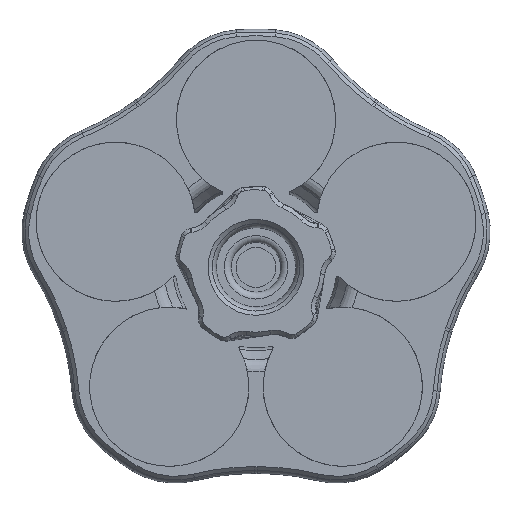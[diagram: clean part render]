
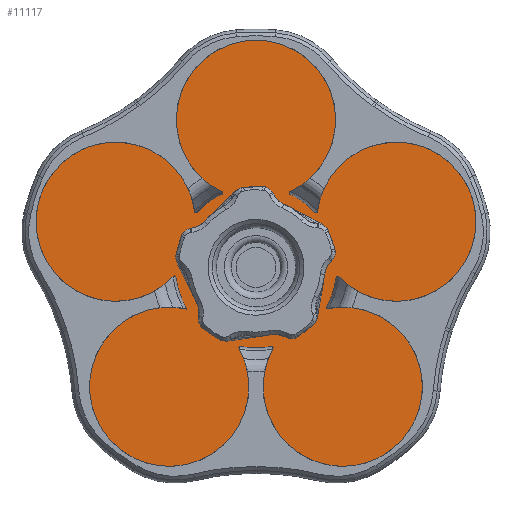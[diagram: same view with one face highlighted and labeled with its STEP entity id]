
A CAD part, front view. The second image highlights one B-rep face of the part: STEP entity #11117.
In plain terms, the highlighted planar face has unit normal (0, -1, 0).
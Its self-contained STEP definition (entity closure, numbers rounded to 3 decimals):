
#48=FACE_BOUND('',#3293,.T.);
#1013=CIRCLE('',#11928,0.1);
#1017=CIRCLE('',#11933,5.775);
#1022=CIRCLE('',#11940,0.1);
#1023=CIRCLE('',#11942,5.775);
#1027=CIRCLE('',#11947,0.1);
#1029=CIRCLE('',#11950,0.1);
#1031=CIRCLE('',#11953,5.85);
#1038=CIRCLE('',#11964,5.775);
#1046=CIRCLE('',#11981,5.775);
#1050=CIRCLE('',#11986,0.1);
#1054=CIRCLE('',#11992,0.1);
#1060=CIRCLE('',#12003,0.1);
#1062=CIRCLE('',#12006,5.85);
#1064=CIRCLE('',#12009,0.1);
#1069=CIRCLE('',#12016,0.1);
#1071=CIRCLE('',#12019,5.775);
#1277=CIRCLE('',#12376,4.65);
#1281=CIRCLE('',#12384,5.85);
#1284=CIRCLE('',#12391,5.85);
#1286=CIRCLE('',#12395,5.85);
#2554=FACE_OUTER_BOUND('',#3292,.T.);
#3292=EDGE_LOOP('',(#9654,#9655,#9656,#9657,#9658,#9659,#9660,#9661,#9662,
#9663,#9664,#9665,#9666,#9667,#9668,#9669,#9670,#9671,#9672));
#3293=EDGE_LOOP('',(#9673));
#4805=VERTEX_POINT('',#22344);
#4806=VERTEX_POINT('',#22346);
#4822=VERTEX_POINT('',#22420);
#4826=VERTEX_POINT('',#22432);
#4827=VERTEX_POINT('',#22434);
#4828=VERTEX_POINT('',#22438);
#4844=VERTEX_POINT('',#22512);
#4847=VERTEX_POINT('',#22519);
#4848=VERTEX_POINT('',#22521);
#4870=VERTEX_POINT('',#22667);
#4889=VERTEX_POINT('',#22814);
#4890=VERTEX_POINT('',#22816);
#4902=VERTEX_POINT('',#22872);
#4904=VERTEX_POINT('',#22881);
#4916=VERTEX_POINT('',#22952);
#4917=VERTEX_POINT('',#22954);
#4919=VERTEX_POINT('',#22963);
#4923=VERTEX_POINT('',#22975);
#4924=VERTEX_POINT('',#22977);
#5091=VERTEX_POINT('',#23862);
#6151=EDGE_CURVE('',#4805,#4806,#1013,.F.);
#6169=EDGE_CURVE('',#4805,#4822,#1017,.T.);
#6175=EDGE_CURVE('',#4826,#4827,#1022,.F.);
#6177=EDGE_CURVE('',#4828,#4827,#1023,.T.);
#6195=EDGE_CURVE('',#4844,#4822,#1027,.F.);
#6198=EDGE_CURVE('',#4847,#4848,#1029,.F.);
#6201=EDGE_CURVE('',#4848,#4844,#1031,.T.);
#6229=EDGE_CURVE('',#4847,#4870,#1038,.T.);
#6258=EDGE_CURVE('',#4890,#4889,#1046,.T.);
#6272=EDGE_CURVE('',#4902,#4889,#1050,.F.);
#6277=EDGE_CURVE('',#4904,#4870,#1054,.F.);
#6293=EDGE_CURVE('',#4916,#4917,#1060,.F.);
#6296=EDGE_CURVE('',#4917,#4904,#1062,.T.);
#6298=EDGE_CURVE('',#4890,#4919,#1064,.F.);
#6305=EDGE_CURVE('',#4923,#4924,#1069,.F.);
#6316=EDGE_CURVE('',#4916,#4924,#1071,.T.);
#6640=EDGE_CURVE('',#5091,#5091,#1277,.T.);
#6644=EDGE_CURVE('',#4806,#4826,#1281,.T.);
#6647=EDGE_CURVE('',#4828,#4902,#1284,.T.);
#6649=EDGE_CURVE('',#4919,#4923,#1286,.T.);
#9654=ORIENTED_EDGE('',*,*,#6229,.T.);
#9655=ORIENTED_EDGE('',*,*,#6277,.F.);
#9656=ORIENTED_EDGE('',*,*,#6296,.F.);
#9657=ORIENTED_EDGE('',*,*,#6293,.F.);
#9658=ORIENTED_EDGE('',*,*,#6316,.T.);
#9659=ORIENTED_EDGE('',*,*,#6305,.F.);
#9660=ORIENTED_EDGE('',*,*,#6649,.F.);
#9661=ORIENTED_EDGE('',*,*,#6298,.F.);
#9662=ORIENTED_EDGE('',*,*,#6258,.T.);
#9663=ORIENTED_EDGE('',*,*,#6272,.F.);
#9664=ORIENTED_EDGE('',*,*,#6647,.F.);
#9665=ORIENTED_EDGE('',*,*,#6177,.T.);
#9666=ORIENTED_EDGE('',*,*,#6175,.F.);
#9667=ORIENTED_EDGE('',*,*,#6644,.F.);
#9668=ORIENTED_EDGE('',*,*,#6151,.F.);
#9669=ORIENTED_EDGE('',*,*,#6169,.T.);
#9670=ORIENTED_EDGE('',*,*,#6195,.F.);
#9671=ORIENTED_EDGE('',*,*,#6201,.F.);
#9672=ORIENTED_EDGE('',*,*,#6198,.F.);
#9673=ORIENTED_EDGE('',*,*,#6640,.F.);
#10533=PLANE('',#12403);
#11117=ADVANCED_FACE('',(#2554,#48),#10533,.T.);
#11928=AXIS2_PLACEMENT_3D('',#22347,#14011,#14012);
#11933=AXIS2_PLACEMENT_3D('',#22422,#14027,#14028);
#11940=AXIS2_PLACEMENT_3D('',#22435,#14042,#14043);
#11942=AXIS2_PLACEMENT_3D('',#22439,#14047,#14048);
#11947=AXIS2_PLACEMENT_3D('',#22514,#14063,#14064);
#11950=AXIS2_PLACEMENT_3D('',#22522,#14070,#14071);
#11953=AXIS2_PLACEMENT_3D('',#22526,#14077,#14078);
#11964=AXIS2_PLACEMENT_3D('',#22669,#14106,#14107);
#11981=AXIS2_PLACEMENT_3D('',#22817,#14147,#14148);
#11986=AXIS2_PLACEMENT_3D('',#22874,#14161,#14162);
#11992=AXIS2_PLACEMENT_3D('',#22883,#14174,#14175);
#12003=AXIS2_PLACEMENT_3D('',#22955,#14200,#14201);
#12006=AXIS2_PLACEMENT_3D('',#22959,#14207,#14208);
#12009=AXIS2_PLACEMENT_3D('',#22964,#14213,#14214);
#12016=AXIS2_PLACEMENT_3D('',#22978,#14229,#14230);
#12019=AXIS2_PLACEMENT_3D('',#23030,#14238,#14239);
#12376=AXIS2_PLACEMENT_3D('',#23864,#15058,#15059);
#12384=AXIS2_PLACEMENT_3D('',#23881,#15074,#15075);
#12391=AXIS2_PLACEMENT_3D('',#23897,#15088,#15089);
#12395=AXIS2_PLACEMENT_3D('',#23910,#15096,#15097);
#12403=AXIS2_PLACEMENT_3D('',#23927,#15112,#15113);
#14011=DIRECTION('center_axis',(0.,1.,0.));
#14012=DIRECTION('ref_axis',(0.807,0.,0.59));
#14027=DIRECTION('center_axis',(0.,-1.,0.));
#14028=DIRECTION('ref_axis',(1.,0.,0.));
#14042=DIRECTION('center_axis',(0.,1.,0.));
#14043=DIRECTION('ref_axis',(-0.807,0.,0.59));
#14047=DIRECTION('center_axis',(0.,-1.,0.));
#14048=DIRECTION('ref_axis',(1.,0.,0.));
#14063=DIRECTION('center_axis',(0.,1.,0.));
#14064=DIRECTION('ref_axis',(-0.811,0.,-0.585));
#14070=DIRECTION('center_axis',(0.,1.,0.));
#14071=DIRECTION('ref_axis',(-0.312,0.,0.95));
#14077=DIRECTION('center_axis',(0.,1.,0.));
#14078=DIRECTION('ref_axis',(1.,0.,0.));
#14106=DIRECTION('center_axis',(0.,-1.,0.));
#14107=DIRECTION('ref_axis',(1.,0.,0.));
#14147=DIRECTION('center_axis',(0.,-1.,0.));
#14148=DIRECTION('ref_axis',(1.,0.,0.));
#14161=DIRECTION('center_axis',(0.,1.,0.));
#14162=DIRECTION('ref_axis',(0.312,0.,0.95));
#14174=DIRECTION('center_axis',(0.,1.,0.));
#14175=DIRECTION('ref_axis',(0.306,0.,-0.952));
#14200=DIRECTION('center_axis',(0.,1.,0.));
#14201=DIRECTION('ref_axis',(-1.,0.,-0.003));
#14207=DIRECTION('center_axis',(0.,1.,0.));
#14208=DIRECTION('ref_axis',(1.,0.,0.));
#14213=DIRECTION('center_axis',(0.,1.,0.));
#14214=DIRECTION('ref_axis',(-0.306,0.,-0.952));
#14229=DIRECTION('center_axis',(0.,1.,0.));
#14230=DIRECTION('ref_axis',(1.,0.,-0.003));
#14238=DIRECTION('center_axis',(0.,-1.,0.));
#14239=DIRECTION('ref_axis',(1.,0.,0.));
#15058=DIRECTION('center_axis',(0.,-1.,0.));
#15059=DIRECTION('ref_axis',(1.,0.,0.));
#15074=DIRECTION('center_axis',(0.,1.,0.));
#15075=DIRECTION('ref_axis',(1.,0.,0.));
#15088=DIRECTION('center_axis',(0.,1.,0.));
#15089=DIRECTION('ref_axis',(1.,0.,0.));
#15096=DIRECTION('center_axis',(0.,1.,0.));
#15097=DIRECTION('ref_axis',(1.,0.,0.));
#15112=DIRECTION('center_axis',(0.,-1.,0.));
#15113=DIRECTION('ref_axis',(1.,0.,0.));
#22344=CARTESIAN_POINT('',(-120.079,-29.7,-5.889));
#22346=CARTESIAN_POINT('',(-120.186,-29.7,-5.743));
#22347=CARTESIAN_POINT('Origin',(-120.167,-29.7,-5.841));
#22420=CARTESIAN_POINT('',(-116.076,-29.7,-2.981));
#22422=CARTESIAN_POINT('Origin',(-115.011,-29.7,-8.656));
#22432=CARTESIAN_POINT('',(-122.414,-29.7,-5.743));
#22434=CARTESIAN_POINT('',(-122.521,-29.7,-5.889));
#22435=CARTESIAN_POINT('Origin',(-122.433,-29.7,-5.841));
#22438=CARTESIAN_POINT('',(-126.307,-29.7,-3.026));
#22439=CARTESIAN_POINT('Origin',(-127.589,-29.7,-8.656));
#22512=CARTESIAN_POINT('',(-116.182,-29.7,-2.834));
#22514=CARTESIAN_POINT('Origin',(-116.095,-29.7,-2.882));
#22519=CARTESIAN_POINT('',(-115.322,-29.7,-0.659));
#22521=CARTESIAN_POINT('',(-115.494,-29.7,-0.715));
#22522=CARTESIAN_POINT('Origin',(-115.395,-29.7,-0.728));
#22526=CARTESIAN_POINT('Origin',(-121.3,-29.7,0.));
#22667=CARTESIAN_POINT('',(-116.851,-29.7,4.047));
#22669=CARTESIAN_POINT('Origin',(-111.124,-29.7,3.306));
#22814=CARTESIAN_POINT('',(-127.278,-29.7,-0.659));
#22816=CARTESIAN_POINT('',(-125.749,-29.7,4.047));
#22817=CARTESIAN_POINT('Origin',(-131.476,-29.7,3.306));
#22872=CARTESIAN_POINT('',(-127.106,-29.7,-0.715));
#22874=CARTESIAN_POINT('Origin',(-127.205,-29.7,-0.728));
#22881=CARTESIAN_POINT('',(-117.023,-29.7,3.992));
#22883=CARTESIAN_POINT('Origin',(-116.95,-29.7,4.06));
#22952=CARTESIAN_POINT('',(-118.826,-29.7,5.482));
#22954=CARTESIAN_POINT('',(-118.825,-29.7,5.301));
#22955=CARTESIAN_POINT('Origin',(-118.783,-29.7,5.391));
#22959=CARTESIAN_POINT('Origin',(-121.3,-29.7,0.));
#22963=CARTESIAN_POINT('',(-125.577,-29.7,3.992));
#22964=CARTESIAN_POINT('Origin',(-125.65,-29.7,4.06));
#22975=CARTESIAN_POINT('',(-123.775,-29.7,5.301));
#22977=CARTESIAN_POINT('',(-123.774,-29.7,5.482));
#22978=CARTESIAN_POINT('Origin',(-123.817,-29.7,5.391));
#23030=CARTESIAN_POINT('Origin',(-121.3,-29.7,10.7));
#23862=CARTESIAN_POINT('',(-125.95,-29.7,0.));
#23864=CARTESIAN_POINT('Origin',(-121.3,-29.7,0.));
#23881=CARTESIAN_POINT('Origin',(-121.3,-29.7,0.));
#23897=CARTESIAN_POINT('Origin',(-121.3,-29.7,0.));
#23910=CARTESIAN_POINT('Origin',(-121.3,-29.7,0.));
#23927=CARTESIAN_POINT('Origin',(-121.3,-29.7,0.));
